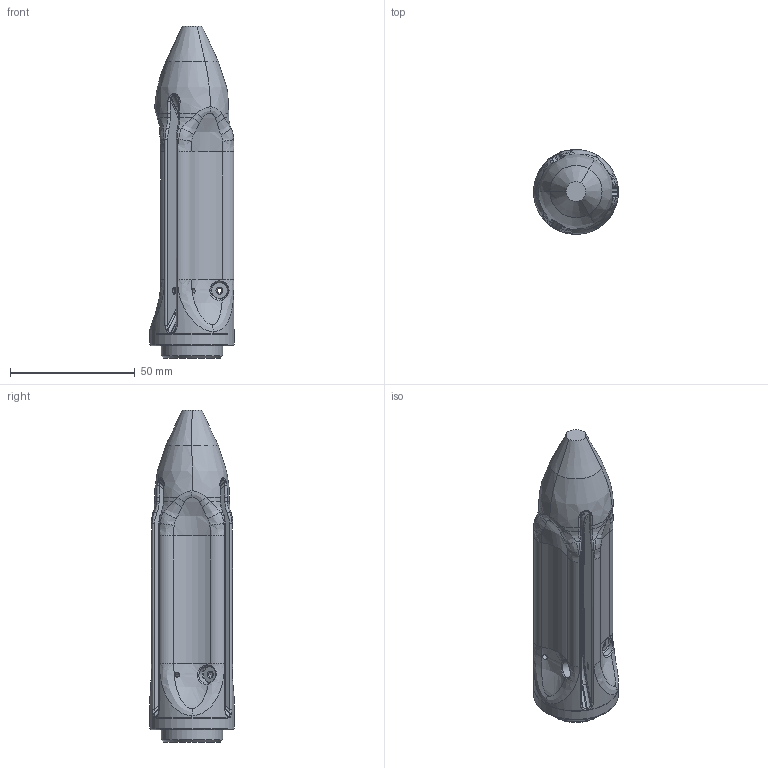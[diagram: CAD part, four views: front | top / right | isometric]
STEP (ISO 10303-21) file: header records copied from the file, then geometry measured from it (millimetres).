
FILE_DESCRIPTION(('FreeCAD Model'),'2;1');
FILE_NAME('Open CASCADE Shape Model','2022-10-05T16:42:01',('Author'),( ''),'Open CASCADE STEP processor 7.6','FreeCAD','Unknown');
FILE_SCHEMA(('AUTOMOTIVE_DESIGN { 1 0 10303 214 1 1 1 1 }'));
Products named in the file (1): Projectile
Bounding box: 34 x 34 x 133 mm (x, y, z)
Volume: 65583.5 mm3; surface area: 19283.1 mm2
Topology: 1 solids, 1 shells, 316 faces, 728 edges, 415 vertices
Faces by surface type: bspline 144, cylinder 88, plane 39, cone 33, torus 12
Full cylindrical faces by diameter (mm): 2 x6, 7 x3, 24.5 x1, 34 x1
Entity records: 50365 total; most frequent: CARTESIAN_POINT 38581, ORIENTED_EDGE 1456, PCURVE 1456, DEFINITIONAL_REPRESENTATION 1456, DIRECTION 1447, LINE 826, VECTOR 826, B_SPLINE_CURVE_WITH_KNOTS 808
